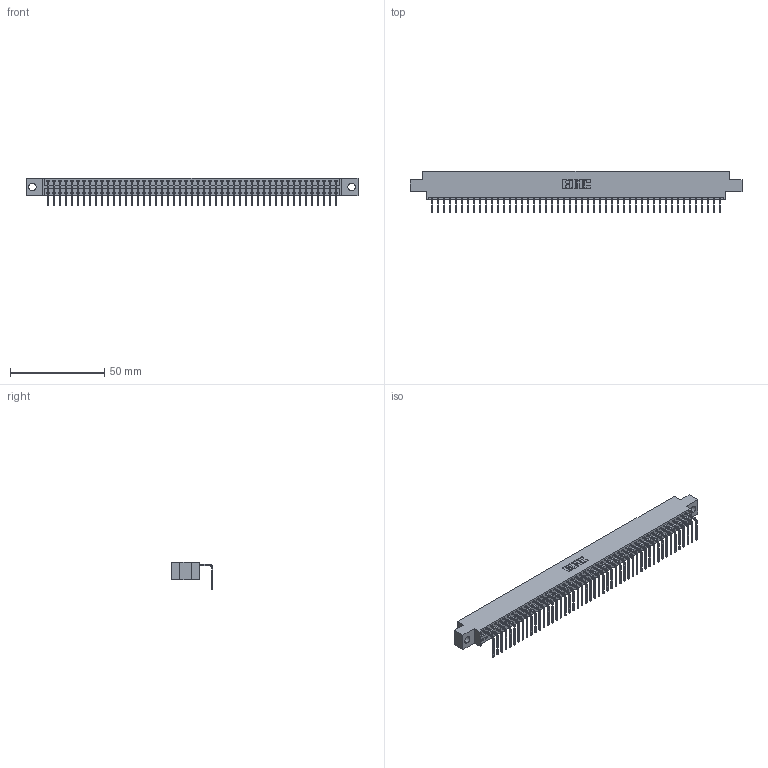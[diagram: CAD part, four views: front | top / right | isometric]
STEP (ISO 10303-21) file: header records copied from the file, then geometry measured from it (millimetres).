
FILE_DESCRIPTION (( 'STEP AP203' ), '1' );
FILE_NAME ('346-049-558-604.STEP', '2022-05-10T02:07:13', ( '' ), ( '' ), 'SwSTEP 2.0', 'SolidWorks 2020', '' );
FILE_SCHEMA (( 'CONFIG_CONTROL_DESIGN' ));
Length unit declared in the file: inch
Products named in the file (3): 346 Part_0.170 Offset - 0.156 Dia-TH; 346-049-558-604; 345-292-001_558 Tail - 2
Assembly tree (50 placements, depth 2):
  346-049-558-604
    346 Part_0.170 Offset - 0.156 Dia-TH
    345-292-001_558 Tail - 2  x49
Bounding box: 176.15 x 22.16 x 14.73 mm (x, y, z)
Volume: 16812.3 mm3; surface area: 22060.3 mm2
Topology: 50 solids, 50 shells, 3080 faces, 9295 edges, 6130 vertices
Faces by surface type: plane 2152, cylinder 928
Entity records: 30103 total; most frequent: CARTESIAN_POINT 5169, ORIENTED_EDGE 5150, DIRECTION 4549, EDGE_CURVE 2575, VECTOR 2247, LINE 2247, VERTEX_POINT 1714, AXIS2_PLACEMENT_3D 1151
